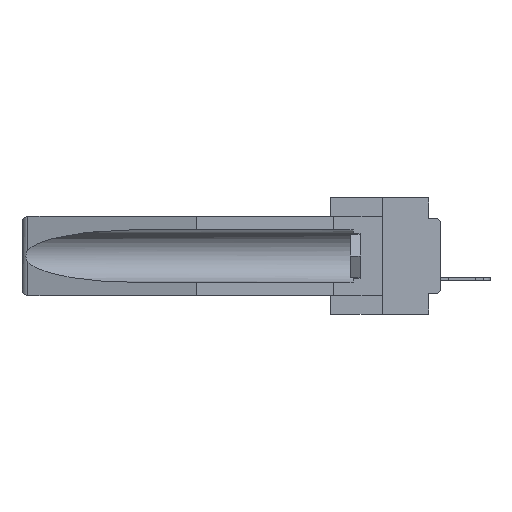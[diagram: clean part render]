
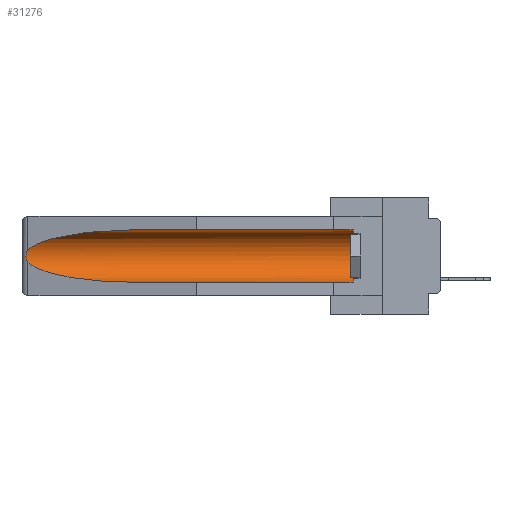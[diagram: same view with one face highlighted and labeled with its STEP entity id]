
A CAD part, left-side view. The second image highlights one B-rep face of the part: STEP entity #31276.
In plain terms, the highlighted cylindrical face has radius 2.857 mm (diameter 5.715 mm), a partial arc.
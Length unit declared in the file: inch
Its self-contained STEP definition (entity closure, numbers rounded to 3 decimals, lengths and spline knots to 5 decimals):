
#113 = B_SPLINE_CURVE_WITH_KNOTS ( 'NONE', 3,
 ( #22820, #28013, #23139, #20449, #12937, #30456, #8178, #15718, #5924, #5598 ),
 .UNSPECIFIED., .F., .F.,
 ( 4, 2, 2, 2, 4 ),
 ( 0., 0.00029, 0.00058, 0.00087, 0.00117 ),
 .UNSPECIFIED. ) ;
#263 = VECTOR ( 'NONE', #24371, 39.37008 ) ;
#1690 = CARTESIAN_POINT ( 'NONE',  ( 0.155, 1.07973, -0.284 ) ) ;
#2313 = FACE_OUTER_BOUND ( 'NONE', #25853, .T. ) ;
#2685 = DIRECTION ( 'NONE',  ( 0., -1., 0. ) ) ;
#3400 = CARTESIAN_POINT ( 'NONE',  ( 0.155, 1.07973, -0.059 ) ) ;
#5168 = LINE ( 'NONE', #23022, #15579 ) ;
#5598 = CARTESIAN_POINT ( 'NONE',  ( 0.26537, 1.52718, -0.19328 ) ) ;
#5924 = CARTESIAN_POINT ( 'NONE',  ( 0.26597, 1.5296, -0.19026 ) ) ;
#6349 = VERTEX_POINT ( 'NONE', #18167 ) ;
#7713 = ORIENTED_EDGE ( 'NONE', *, *, #25716, .T. ) ;
#8178 = CARTESIAN_POINT ( 'NONE',  ( 0.2673, 1.53269, -0.17917 ) ) ;
#8222 = ORIENTED_EDGE ( 'NONE', *, *, #8244, .F. ) ;
#8244 = EDGE_CURVE ( 'NONE', #27780, #18098, #5168, .T. ) ;
#9820 = CARTESIAN_POINT ( 'NONE',  ( 0.155, 0.126, -0.059 ) ) ;
#10785 =( BOUNDED_CURVE ( )  B_SPLINE_CURVE ( 3, ( #3400, #20611, #28059, #25447 ),
 .UNSPECIFIED., .F., .F. ) 
 B_SPLINE_CURVE_WITH_KNOTS ( ( 4, 4 ),
 ( 4.71239, 6.08839 ),
 .UNSPECIFIED. ) 
 CURVE ( )  GEOMETRIC_REPRESENTATION_ITEM ( )  RATIONAL_B_SPLINE_CURVE ( ( 1., 0.848, 0.848, 1. ) ) 
 REPRESENTATION_ITEM ( '' )  );
#11332 = VERTEX_POINT ( 'NONE', #23176 ) ;
#11694 = VERTEX_POINT ( 'NONE', #21092 ) ;
#12318 = CYLINDRICAL_SURFACE ( 'NONE', #15465, 0.1125 ) ;
#12937 = CARTESIAN_POINT ( 'NONE',  ( 0.2675, 1.53308, -0.16763 ) ) ;
#13792 = DIRECTION ( 'NONE',  ( 0., 1., 0. ) ) ;
#13886 = EDGE_CURVE ( 'NONE', #6349, #18098, #25995, .T. ) ;
#13984 = EDGE_CURVE ( 'NONE', #11694, #11332, #10785, .T. ) ;
#14334 = EDGE_CURVE ( 'NONE', #29650, #11694, #22251, .T. ) ;
#14674 = CARTESIAN_POINT ( 'NONE',  ( 0.155, 0.126, -0.284 ) ) ;
#14745 = CARTESIAN_POINT ( 'NONE',  ( 0.155, 0.126, -0.1715 ) ) ;
#15036 = DIRECTION ( 'NONE',  ( 0., 1., 0. ) ) ;
#15465 = AXIS2_PLACEMENT_3D ( 'NONE', #25035, #15036, #27349 ) ;
#15579 = VECTOR ( 'NONE', #13792, 39.37008 ) ;
#15718 = CARTESIAN_POINT ( 'NONE',  ( 0.26655, 1.53094, -0.18657 ) ) ;
#17900 = AXIS2_PLACEMENT_3D ( 'NONE', #14745, #2685, #27030 ) ;
#18098 = VERTEX_POINT ( 'NONE', #1690 ) ;
#18167 = CARTESIAN_POINT ( 'NONE',  ( 0.26537, 1.52718, -0.19328 ) ) ;
#18803 = ORIENTED_EDGE ( 'NONE', *, *, #13886, .T. ) ;
#19772 = EDGE_CURVE ( 'NONE', #27780, #29650, #25047, .T. ) ;
#20273 = CARTESIAN_POINT ( 'NONE',  ( 0.155, 1.07973, -0.284 ) ) ;
#20449 = CARTESIAN_POINT ( 'NONE',  ( 0.2673, 1.5327, -0.16383 ) ) ;
#20611 = CARTESIAN_POINT ( 'NONE',  ( 0.21114, 1.30732, -0.059 ) ) ;
#21092 = CARTESIAN_POINT ( 'NONE',  ( 0.155, 1.07973, -0.059 ) ) ;
#21506 = ORIENTED_EDGE ( 'NONE', *, *, #19772, .T. ) ;
#21803 = CARTESIAN_POINT ( 'NONE',  ( 0.155, -0.30754, -0.059 ) ) ;
#22251 = LINE ( 'NONE', #21803, #263 ) ;
#22317 = ORIENTED_EDGE ( 'NONE', *, *, #14334, .T. ) ;
#22820 = CARTESIAN_POINT ( 'NONE',  ( 0.26537, 1.52718, -0.14972 ) ) ;
#23022 = CARTESIAN_POINT ( 'NONE',  ( 0.155, -0.30754, -0.284 ) ) ;
#23139 = CARTESIAN_POINT ( 'NONE',  ( 0.26654, 1.53092, -0.15636 ) ) ;
#23176 = CARTESIAN_POINT ( 'NONE',  ( 0.26537, 1.52718, -0.14972 ) ) ;
#23564 = ORIENTED_EDGE ( 'NONE', *, *, #13984, .T. ) ;
#24371 = DIRECTION ( 'NONE',  ( 0., 1., 0. ) ) ;
#25006 = CARTESIAN_POINT ( 'NONE',  ( 0.25451, 1.48313, -0.24835 ) ) ;
#25035 = CARTESIAN_POINT ( 'NONE',  ( 0.155, -0.30754, -0.1715 ) ) ;
#25047 = CIRCLE ( 'NONE', #17900, 0.1125 ) ;
#25234 = CARTESIAN_POINT ( 'NONE',  ( 0.26537, 1.52718, -0.19328 ) ) ;
#25447 = CARTESIAN_POINT ( 'NONE',  ( 0.26537, 1.52718, -0.14972 ) ) ;
#25716 = EDGE_CURVE ( 'NONE', #11332, #6349, #113, .T. ) ;
#25853 = EDGE_LOOP ( 'NONE', ( #23564, #7713, #18803, #8222, #21506, #22317 ) ) ;
#25995 =( BOUNDED_CURVE ( )  B_SPLINE_CURVE ( 3, ( #25234, #25006, #29965, #20273 ),
 .UNSPECIFIED., .F., .F. ) 
 B_SPLINE_CURVE_WITH_KNOTS ( ( 4, 4 ),
 ( 0.1948, 1.5708 ),
 .UNSPECIFIED. ) 
 CURVE ( )  GEOMETRIC_REPRESENTATION_ITEM ( )  RATIONAL_B_SPLINE_CURVE ( ( 1., 0.848, 0.848, 1. ) ) 
 REPRESENTATION_ITEM ( '' )  );
#27030 = DIRECTION ( 'NONE',  ( 0., 0., 1. ) ) ;
#27349 = DIRECTION ( 'NONE',  ( 0., 0., 1. ) ) ;
#27780 = VERTEX_POINT ( 'NONE', #14674 ) ;
#28013 = CARTESIAN_POINT ( 'NONE',  ( 0.26597, 1.52961, -0.15275 ) ) ;
#28059 = CARTESIAN_POINT ( 'NONE',  ( 0.25451, 1.48313, -0.09465 ) ) ;
#29650 = VERTEX_POINT ( 'NONE', #9820 ) ;
#29965 = CARTESIAN_POINT ( 'NONE',  ( 0.21114, 1.30732, -0.284 ) ) ;
#30456 = CARTESIAN_POINT ( 'NONE',  ( 0.2675, 1.53308, -0.17534 ) ) ;
#31276 = ADVANCED_FACE ( 'NONE', ( #2313 ), #12318, .F. ) ;
